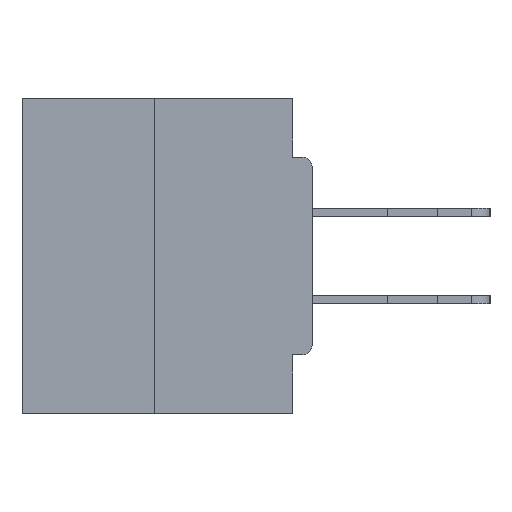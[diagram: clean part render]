
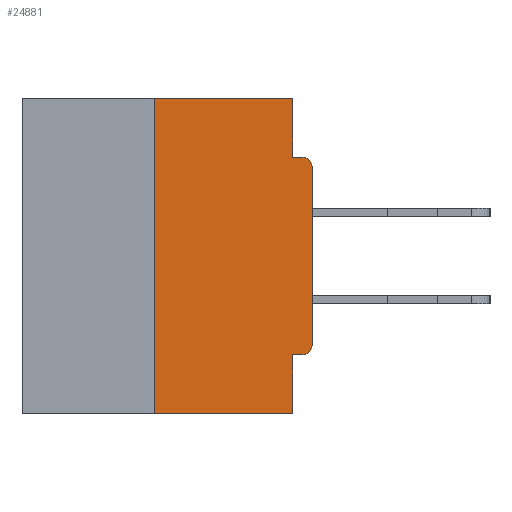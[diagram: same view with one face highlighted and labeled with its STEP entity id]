
A CAD part, left-side view. The second image highlights one B-rep face of the part: STEP entity #24881.
In plain terms, the highlighted planar face has unit normal (-1, 0, 0).
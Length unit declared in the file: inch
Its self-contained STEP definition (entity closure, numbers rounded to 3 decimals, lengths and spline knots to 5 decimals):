
#820 = CARTESIAN_POINT ( 'NONE',  ( 0., 0., -0.3915 ) ) ;
#2569 = ORIENTED_EDGE ( 'NONE', *, *, #13507, .T. ) ;
#3057 = CARTESIAN_POINT ( 'NONE',  ( 0., 0.46, -0.5 ) ) ;
#3351 = CARTESIAN_POINT ( 'NONE',  ( 0., 0.031, -0.5 ) ) ;
#3394 = DIRECTION ( 'NONE',  ( -1., 0., 0. ) ) ;
#3541 = EDGE_CURVE ( 'NONE', #12463, #3626, #30537, .T. ) ;
#3626 = VERTEX_POINT ( 'NONE', #29146 ) ;
#4163 = FACE_OUTER_BOUND ( 'NONE', #16792, .T. ) ;
#4800 = PLANE ( 'NONE',  #8608 ) ;
#5421 = DIRECTION ( 'NONE',  ( 0., -1., 0. ) ) ;
#5424 = VECTOR ( 'NONE', #5421, 39.37008 ) ;
#5426 = DIRECTION ( 'NONE',  ( 0., 0., -1. ) ) ;
#5462 = AXIS2_PLACEMENT_3D ( 'NONE', #39424, #30155, #5426 ) ;
#5560 = CARTESIAN_POINT ( 'NONE',  ( 0., 0.031, 0. ) ) ;
#6230 = VECTOR ( 'NONE', #32391, 39.37008 ) ;
#6614 = CARTESIAN_POINT ( 'NONE',  ( 0., 0., -0.1085 ) ) ;
#6762 = DIRECTION ( 'NONE',  ( 0., 0., 1. ) ) ;
#7109 = VERTEX_POINT ( 'NONE', #32553 ) ;
#7736 = DIRECTION ( 'NONE',  ( 1., 0., 0. ) ) ;
#8294 = DIRECTION ( 'NONE',  ( 0., 1., 0. ) ) ;
#8608 = AXIS2_PLACEMENT_3D ( 'NONE', #35770, #7736, #16868 ) ;
#9060 = VECTOR ( 'NONE', #40905, 39.37008 ) ;
#9218 = VERTEX_POINT ( 'NONE', #3351 ) ;
#10611 = VERTEX_POINT ( 'NONE', #820 ) ;
#10670 = LINE ( 'NONE', #35440, #6230 ) ;
#11406 = CARTESIAN_POINT ( 'NONE',  ( 0., 0.031, 0. ) ) ;
#11445 = EDGE_CURVE ( 'NONE', #33083, #9218, #29837, .T. ) ;
#11753 = AXIS2_PLACEMENT_3D ( 'NONE', #25840, #3394, #38363 ) ;
#12463 = VERTEX_POINT ( 'NONE', #31441 ) ;
#13507 = EDGE_CURVE ( 'NONE', #22183, #7109, #33142, .T. ) ;
#13720 = VERTEX_POINT ( 'NONE', #22910 ) ;
#14811 = CARTESIAN_POINT ( 'NONE',  ( 0., 0.031, -0.4065 ) ) ;
#16792 = EDGE_LOOP ( 'NONE', ( #26192, #17016, #20711, #25823, #21116, #33231, #34517, #2569, #33053, #34586 ) ) ;
#16868 = DIRECTION ( 'NONE',  ( 0., 0., -1. ) ) ;
#17016 = ORIENTED_EDGE ( 'NONE', *, *, #3541, .F. ) ;
#17432 = CARTESIAN_POINT ( 'NONE',  ( 0., 0.46, 0. ) ) ;
#18220 = VECTOR ( 'NONE', #8294, 39.37008 ) ;
#19643 = CARTESIAN_POINT ( 'NONE',  ( 0., 0.031, -0.0935 ) ) ;
#20711 = ORIENTED_EDGE ( 'NONE', *, *, #32487, .T. ) ;
#20811 = CARTESIAN_POINT ( 'NONE',  ( 0., 0.031, -0.5 ) ) ;
#21092 = DIRECTION ( 'NONE',  ( 0., 0., -1. ) ) ;
#21116 = ORIENTED_EDGE ( 'NONE', *, *, #35728, .F. ) ;
#21465 = VECTOR ( 'NONE', #21092, 39.37008 ) ;
#22183 = VERTEX_POINT ( 'NONE', #6614 ) ;
#22910 = CARTESIAN_POINT ( 'NONE',  ( 0., 0.015, -0.4065 ) ) ;
#23884 = EDGE_CURVE ( 'NONE', #10611, #22183, #10670, .T. ) ;
#24163 = DIRECTION ( 'NONE',  ( 0., 0., -1. ) ) ;
#24881 = ADVANCED_FACE ( 'NONE', ( #4163 ), #4800, .F. ) ;
#25189 = LINE ( 'NONE', #29983, #18220 ) ;
#25823 = ORIENTED_EDGE ( 'NONE', *, *, #11445, .F. ) ;
#25840 = CARTESIAN_POINT ( 'NONE',  ( 0., 0.015, -0.1085 ) ) ;
#26192 = ORIENTED_EDGE ( 'NONE', *, *, #28632, .F. ) ;
#27935 = EDGE_CURVE ( 'NONE', #32672, #7109, #39515, .T. ) ;
#28632 = EDGE_CURVE ( 'NONE', #3626, #29559, #35997, .T. ) ;
#29146 = CARTESIAN_POINT ( 'NONE',  ( 0., 0.25, 0. ) ) ;
#29559 = VERTEX_POINT ( 'NONE', #5560 ) ;
#29837 = LINE ( 'NONE', #20811, #21465 ) ;
#29979 = LINE ( 'NONE', #11406, #32955 ) ;
#29983 = CARTESIAN_POINT ( 'NONE',  ( 0., 0., -0.4065 ) ) ;
#30155 = DIRECTION ( 'NONE',  ( -1., 0., 0. ) ) ;
#30537 = LINE ( 'NONE', #37971, #40391 ) ;
#30716 = CARTESIAN_POINT ( 'NONE',  ( 0., 0., -0.0935 ) ) ;
#31441 = CARTESIAN_POINT ( 'NONE',  ( 0., 0.25, -0.5 ) ) ;
#31798 = LINE ( 'NONE', #3057, #9060 ) ;
#31879 = CIRCLE ( 'NONE', #5462, 0.015 ) ;
#32391 = DIRECTION ( 'NONE',  ( 0., 0., 1. ) ) ;
#32487 = EDGE_CURVE ( 'NONE', #12463, #9218, #31798, .T. ) ;
#32553 = CARTESIAN_POINT ( 'NONE',  ( 0., 0.015, -0.0935 ) ) ;
#32672 = VERTEX_POINT ( 'NONE', #19643 ) ;
#32955 = VECTOR ( 'NONE', #24163, 39.37008 ) ;
#33053 = ORIENTED_EDGE ( 'NONE', *, *, #27935, .F. ) ;
#33083 = VERTEX_POINT ( 'NONE', #14811 ) ;
#33142 = CIRCLE ( 'NONE', #11753, 0.015 ) ;
#33231 = ORIENTED_EDGE ( 'NONE', *, *, #38197, .T. ) ;
#34517 = ORIENTED_EDGE ( 'NONE', *, *, #23884, .T. ) ;
#34586 = ORIENTED_EDGE ( 'NONE', *, *, #37244, .F. ) ;
#35440 = CARTESIAN_POINT ( 'NONE',  ( 0., 0., 0. ) ) ;
#35728 = EDGE_CURVE ( 'NONE', #13720, #33083, #25189, .T. ) ;
#35770 = CARTESIAN_POINT ( 'NONE',  ( 0., 0.46, 0. ) ) ;
#35997 = LINE ( 'NONE', #17432, #38497 ) ;
#36619 = DIRECTION ( 'NONE',  ( 0., -1., 0. ) ) ;
#37244 = EDGE_CURVE ( 'NONE', #29559, #32672, #29979, .T. ) ;
#37971 = CARTESIAN_POINT ( 'NONE',  ( 0., 0.25, 0. ) ) ;
#38197 = EDGE_CURVE ( 'NONE', #13720, #10611, #31879, .T. ) ;
#38363 = DIRECTION ( 'NONE',  ( 0., 0., -1. ) ) ;
#38497 = VECTOR ( 'NONE', #36619, 39.37008 ) ;
#39424 = CARTESIAN_POINT ( 'NONE',  ( 0., 0.015, -0.3915 ) ) ;
#39515 = LINE ( 'NONE', #30716, #5424 ) ;
#40391 = VECTOR ( 'NONE', #6762, 39.37008 ) ;
#40905 = DIRECTION ( 'NONE',  ( 0., -1., 0. ) ) ;
